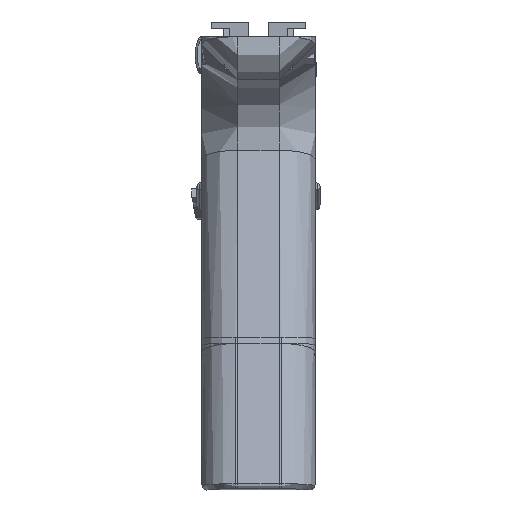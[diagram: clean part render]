
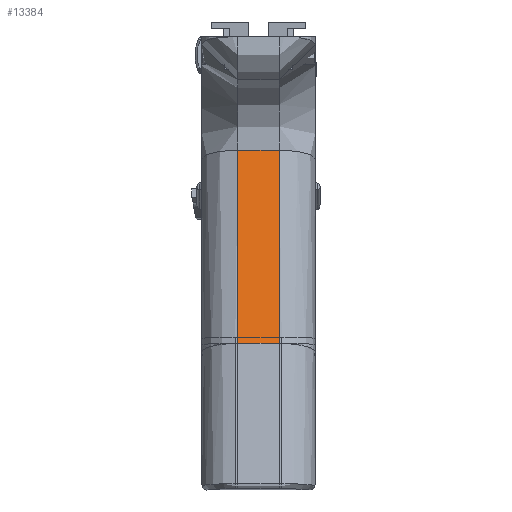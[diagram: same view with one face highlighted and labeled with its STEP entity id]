
A CAD part, front view. The second image highlights one B-rep face of the part: STEP entity #13384.
In plain terms, the highlighted face is planar.
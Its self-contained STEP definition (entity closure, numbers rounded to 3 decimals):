
#1047=PLANE('',#14603);
#1671=FACE_OUTER_BOUND('',#2447,.T.);
#2447=EDGE_LOOP('',(#11608,#11609,#11610,#11611));
#3473=LINE('',#23670,#4668);
#3629=LINE('',#24522,#4824);
#3630=LINE('',#24525,#4825);
#3631=LINE('',#24526,#4826);
#4668=VECTOR('',#17265,10.);
#4824=VECTOR('',#17669,10.);
#4825=VECTOR('',#17672,10.);
#4826=VECTOR('',#17673,10.);
#6284=VERTEX_POINT('',#23666);
#6285=VERTEX_POINT('',#23668);
#6424=VERTEX_POINT('',#24500);
#6427=VERTEX_POINT('',#24524);
#8007=EDGE_CURVE('',#6284,#6285,#3473,.T.);
#8233=EDGE_CURVE('',#6284,#6424,#3629,.T.);
#8234=EDGE_CURVE('',#6427,#6285,#3630,.T.);
#8235=EDGE_CURVE('',#6424,#6427,#3631,.T.);
#11608=ORIENTED_EDGE('',*,*,#8234,.F.);
#11609=ORIENTED_EDGE('',*,*,#8235,.F.);
#11610=ORIENTED_EDGE('',*,*,#8233,.F.);
#11611=ORIENTED_EDGE('',*,*,#8007,.T.);
#13384=ADVANCED_FACE('',(#1671),#1047,.T.);
#14603=AXIS2_PLACEMENT_3D('',#24523,#17670,#17671);
#17265=DIRECTION('',(0.,-0.249,0.969));
#17669=DIRECTION('',(-1.,0.,0.));
#17670=DIRECTION('center_axis',(0.,-0.969,
-0.249));
#17671=DIRECTION('ref_axis',(0.,-0.249,0.969));
#17672=DIRECTION('',(1.,0.,0.));
#17673=DIRECTION('',(0.,-0.249,0.969));
#23666=CARTESIAN_POINT('',(13.45,-71.634,19.877));
#23668=CARTESIAN_POINT('',(13.45,-83.628,66.536));
#23670=CARTESIAN_POINT('',(13.45,-83.554,66.245));
#24500=CARTESIAN_POINT('',(3.45,-71.634,19.877));
#24522=CARTESIAN_POINT('',(22.175,-71.634,19.877));
#24523=CARTESIAN_POINT('Origin',(22.175,-71.634,19.877));
#24524=CARTESIAN_POINT('',(3.45,-83.628,66.536));
#24525=CARTESIAN_POINT('',(22.175,-83.628,66.536));
#24526=CARTESIAN_POINT('',(3.45,-83.554,66.245));
